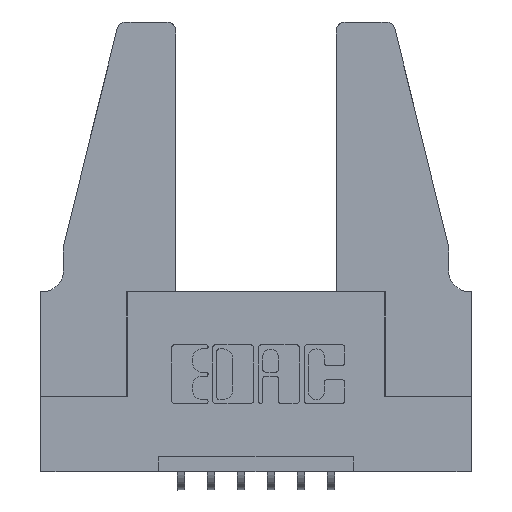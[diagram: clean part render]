
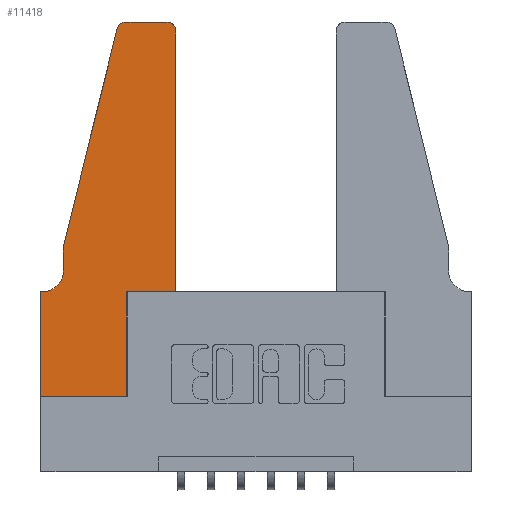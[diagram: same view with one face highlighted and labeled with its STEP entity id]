
A CAD part, top view. The second image highlights one B-rep face of the part: STEP entity #11418.
In plain terms, the highlighted planar face has unit normal (0, 0, 1).
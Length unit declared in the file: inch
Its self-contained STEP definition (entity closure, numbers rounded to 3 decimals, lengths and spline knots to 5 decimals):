
#14 = ORIENTED_EDGE ( 'NONE', *, *, #8578, .T. ) ;
#88 = CARTESIAN_POINT ( 'NONE',  ( 0.0755, 0.5, 0.37 ) ) ;
#316 = DIRECTION ( 'NONE',  ( 0., 0., -1. ) ) ;
#533 = DIRECTION ( 'NONE',  ( 1., 0., 0. ) ) ;
#663 = LINE ( 'NONE', #7208, #11440 ) ;
#673 = CARTESIAN_POINT ( 'NONE',  ( 0.4505, 0.35, 0.37 ) ) ;
#809 = LINE ( 'NONE', #2670, #6845 ) ;
#884 = CARTESIAN_POINT ( 'NONE',  ( 0., 0., 0.37 ) ) ;
#1041 = ORIENTED_EDGE ( 'NONE', *, *, #8770, .T. ) ;
#1542 = EDGE_CURVE ( 'NONE', #7584, #3071, #11116, .T. ) ;
#1641 = LINE ( 'NONE', #9153, #2903 ) ;
#2273 = VERTEX_POINT ( 'NONE', #88 ) ;
#2360 = VECTOR ( 'NONE', #10279, 39.37008 ) ;
#2363 = AXIS2_PLACEMENT_3D ( 'NONE', #5865, #5753, #533 ) ;
#2505 = LINE ( 'NONE', #6730, #6712 ) ;
#2589 = ORIENTED_EDGE ( 'NONE', *, *, #5145, .T. ) ;
#2616 = VERTEX_POINT ( 'NONE', #7223 ) ;
#2636 = CARTESIAN_POINT ( 'NONE',  ( 0.25487, 1.22718, 0.37 ) ) ;
#2658 = EDGE_CURVE ( 'NONE', #4495, #9110, #2667, .T. ) ;
#2667 = CIRCLE ( 'NONE', #2363, 0.03 ) ;
#2670 = CARTESIAN_POINT ( 'NONE',  ( 0.4505, 0.35, 0.37 ) ) ;
#2840 = CARTESIAN_POINT ( 'NONE',  ( 0.2605, 1.25, 0.37 ) ) ;
#2903 = VECTOR ( 'NONE', #3834, 39.37008 ) ;
#2917 = VERTEX_POINT ( 'NONE', #673 ) ;
#3071 = VERTEX_POINT ( 'NONE', #5194 ) ;
#3126 = CARTESIAN_POINT ( 'NONE',  ( 0.2865, 0.35, 0.37 ) ) ;
#3410 = DIRECTION ( 'NONE',  ( -1., 0., 0. ) ) ;
#3431 = VERTEX_POINT ( 'NONE', #10269 ) ;
#3508 = DIRECTION ( 'NONE',  ( 0., 0., 1. ) ) ;
#3834 = DIRECTION ( 'NONE',  ( -0.239, -0.971, 0. ) ) ;
#4370 = DIRECTION ( 'NONE',  ( 1., 0., 0. ) ) ;
#4480 = EDGE_CURVE ( 'NONE', #3431, #2616, #10343, .T. ) ;
#4495 = VERTEX_POINT ( 'NONE', #11390 ) ;
#4499 = AXIS2_PLACEMENT_3D ( 'NONE', #5776, #316, #11083 ) ;
#4650 = EDGE_CURVE ( 'NONE', #3071, #5429, #10613, .T. ) ;
#4692 = EDGE_CURVE ( 'NONE', #2616, #7584, #9079, .T. ) ;
#4783 = DIRECTION ( 'NONE',  ( 0., 1., 0. ) ) ;
#4847 = DIRECTION ( 'NONE',  ( 0., -1., 0. ) ) ;
#4848 = CARTESIAN_POINT ( 'NONE',  ( 0., 0., 0.37 ) ) ;
#4885 = DIRECTION ( 'NONE',  ( 1., 0., 0. ) ) ;
#4943 = EDGE_CURVE ( 'NONE', #8716, #2273, #1641, .T. ) ;
#4948 = EDGE_CURVE ( 'NONE', #9110, #8997, #10888, .T. ) ;
#5130 = CARTESIAN_POINT ( 'NONE',  ( 0.0755, 0.35, 0.37 ) ) ;
#5145 = EDGE_CURVE ( 'NONE', #2917, #4495, #663, .T. ) ;
#5194 = CARTESIAN_POINT ( 'NONE',  ( 0.2865, 0., 0.37 ) ) ;
#5264 = DIRECTION ( 'NONE',  ( 1., 0., 0. ) ) ;
#5429 = VERTEX_POINT ( 'NONE', #7231 ) ;
#5672 = AXIS2_PLACEMENT_3D ( 'NONE', #6934, #9837, #4370 ) ;
#5753 = DIRECTION ( 'NONE',  ( 0., 0., 1. ) ) ;
#5776 = CARTESIAN_POINT ( 'NONE',  ( 0.0055, 0.42, 0.37 ) ) ;
#5865 = CARTESIAN_POINT ( 'NONE',  ( 0.4205, 1.22, 0.37 ) ) ;
#6353 = ORIENTED_EDGE ( 'NONE', *, *, #4650, .T. ) ;
#6510 = VECTOR ( 'NONE', #4885, 39.37008 ) ;
#6653 = ORIENTED_EDGE ( 'NONE', *, *, #4480, .T. ) ;
#6712 = VECTOR ( 'NONE', #4847, 39.37008 ) ;
#6730 = CARTESIAN_POINT ( 'NONE',  ( 0.0755, 0.5, 0.37 ) ) ;
#6845 = VECTOR ( 'NONE', #8947, 39.37008 ) ;
#6934 = CARTESIAN_POINT ( 'NONE',  ( 0., 0.35, 0.37 ) ) ;
#6935 = CIRCLE ( 'NONE', #11434, 0.03 ) ;
#7025 = CARTESIAN_POINT ( 'NONE',  ( 0.284, 1.22, 0.37 ) ) ;
#7174 = ORIENTED_EDGE ( 'NONE', *, *, #4692, .T. ) ;
#7208 = CARTESIAN_POINT ( 'NONE',  ( 0.4505, 0.35, 0.37 ) ) ;
#7223 = CARTESIAN_POINT ( 'NONE',  ( 0., 0.35, 0.37 ) ) ;
#7231 = CARTESIAN_POINT ( 'NONE',  ( 0.2865, 0.35, 0.37 ) ) ;
#7394 = EDGE_LOOP ( 'NONE', ( #7602, #9855, #10989, #1041, #14, #6653, #7174, #8262, #6353, #10115, #2589, #7880 ) ) ;
#7584 = VERTEX_POINT ( 'NONE', #884 ) ;
#7602 = ORIENTED_EDGE ( 'NONE', *, *, #4948, .T. ) ;
#7880 = ORIENTED_EDGE ( 'NONE', *, *, #2658, .T. ) ;
#8219 = VECTOR ( 'NONE', #11101, 39.37008 ) ;
#8262 = ORIENTED_EDGE ( 'NONE', *, *, #1542, .T. ) ;
#8394 = CARTESIAN_POINT ( 'NONE',  ( 0.284, 1.25, 0.37 ) ) ;
#8578 = EDGE_CURVE ( 'NONE', #10196, #3431, #10091, .T. ) ;
#8710 = PLANE ( 'NONE',  #5672 ) ;
#8716 = VERTEX_POINT ( 'NONE', #2636 ) ;
#8770 = EDGE_CURVE ( 'NONE', #2273, #10196, #2505, .T. ) ;
#8947 = DIRECTION ( 'NONE',  ( 1., 0., 0. ) ) ;
#8997 = VERTEX_POINT ( 'NONE', #8394 ) ;
#9079 = LINE ( 'NONE', #11066, #8219 ) ;
#9110 = VERTEX_POINT ( 'NONE', #11592 ) ;
#9153 = CARTESIAN_POINT ( 'NONE',  ( 0.0755, 0.5, 0.37 ) ) ;
#9217 = EDGE_CURVE ( 'NONE', #5429, #2917, #809, .T. ) ;
#9513 = VECTOR ( 'NONE', #3410, 39.37008 ) ;
#9837 = DIRECTION ( 'NONE',  ( 0., 0., 1. ) ) ;
#9855 = ORIENTED_EDGE ( 'NONE', *, *, #11278, .T. ) ;
#9990 = CARTESIAN_POINT ( 'NONE',  ( 0.0755, 0.42, 0.37 ) ) ;
#10060 = VECTOR ( 'NONE', #10981, 39.37008 ) ;
#10091 = CIRCLE ( 'NONE', #4499, 0.07 ) ;
#10115 = ORIENTED_EDGE ( 'NONE', *, *, #9217, .T. ) ;
#10196 = VERTEX_POINT ( 'NONE', #9990 ) ;
#10269 = CARTESIAN_POINT ( 'NONE',  ( 0.0055, 0.35, 0.37 ) ) ;
#10279 = DIRECTION ( 'NONE',  ( 0., 1., 0. ) ) ;
#10343 = LINE ( 'NONE', #5130, #9513 ) ;
#10613 = LINE ( 'NONE', #3126, #2360 ) ;
#10888 = LINE ( 'NONE', #2840, #10060 ) ;
#10981 = DIRECTION ( 'NONE',  ( -1., 0., 0. ) ) ;
#10989 = ORIENTED_EDGE ( 'NONE', *, *, #4943, .T. ) ;
#11066 = CARTESIAN_POINT ( 'NONE',  ( 0., 0., 0.37 ) ) ;
#11083 = DIRECTION ( 'NONE',  ( -1., 0., 0. ) ) ;
#11101 = DIRECTION ( 'NONE',  ( 0., -1., 0. ) ) ;
#11116 = LINE ( 'NONE', #4848, #6510 ) ;
#11278 = EDGE_CURVE ( 'NONE', #8997, #8716, #6935, .T. ) ;
#11286 = FACE_OUTER_BOUND ( 'NONE', #7394, .T. ) ;
#11390 = CARTESIAN_POINT ( 'NONE',  ( 0.4505, 1.22, 0.37 ) ) ;
#11418 = ADVANCED_FACE ( 'NONE', ( #11286 ), #8710, .T. ) ;
#11434 = AXIS2_PLACEMENT_3D ( 'NONE', #7025, #3508, #5264 ) ;
#11440 = VECTOR ( 'NONE', #4783, 39.37008 ) ;
#11592 = CARTESIAN_POINT ( 'NONE',  ( 0.4205, 1.25, 0.37 ) ) ;
